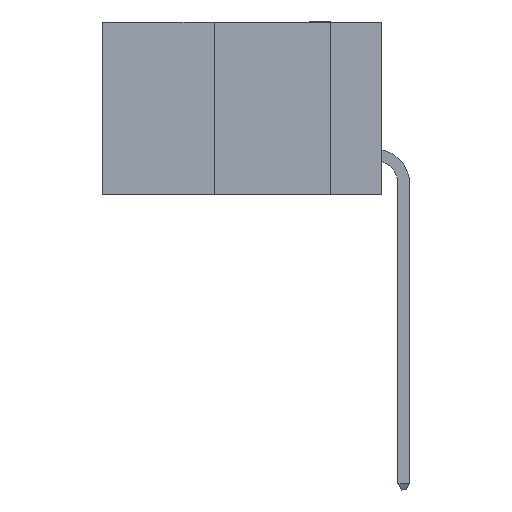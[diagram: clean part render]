
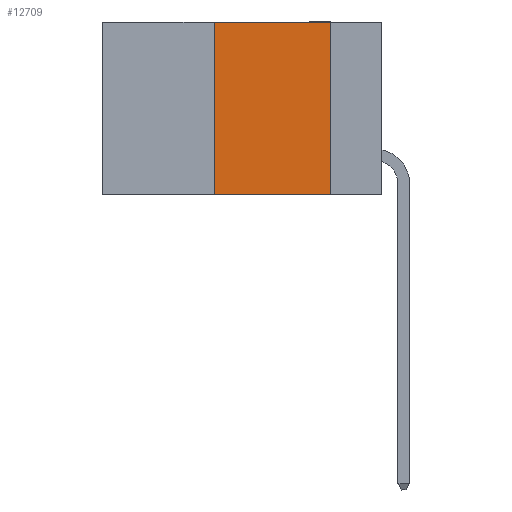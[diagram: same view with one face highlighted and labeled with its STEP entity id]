
A CAD part, left-side view. The second image highlights one B-rep face of the part: STEP entity #12709.
In plain terms, the highlighted planar face has unit normal (-1, 0, 0).
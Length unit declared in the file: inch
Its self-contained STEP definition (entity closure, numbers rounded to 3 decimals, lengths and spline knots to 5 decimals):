
#1251 = DIRECTION ( 'NONE',  ( 0., 0., -1. ) ) ;
#2239 = CARTESIAN_POINT ( 'NONE',  ( 0., 0.36, 0. ) ) ;
#2741 = DIRECTION ( 'NONE',  ( 1., 0., 0. ) ) ;
#4065 = CARTESIAN_POINT ( 'NONE',  ( 0., 0.11, 0. ) ) ;
#4241 = DIRECTION ( 'NONE',  ( 0., 0., 1. ) ) ;
#4516 = VERTEX_POINT ( 'NONE', #2239 ) ;
#4524 = ORIENTED_EDGE ( 'NONE', *, *, #6573, .F. ) ;
#4601 = EDGE_LOOP ( 'NONE', ( #8562, #8149, #4524, #5804 ) ) ;
#5652 = EDGE_CURVE ( 'NONE', #10325, #14951, #13583, .T. ) ;
#5702 = CARTESIAN_POINT ( 'NONE',  ( 0., 0.36, -0.37 ) ) ;
#5804 = ORIENTED_EDGE ( 'NONE', *, *, #5652, .T. ) ;
#5971 = LINE ( 'NONE', #6928, #12711 ) ;
#6346 = CARTESIAN_POINT ( 'NONE',  ( 0., 0.6, -0.37 ) ) ;
#6573 = EDGE_CURVE ( 'NONE', #10325, #4516, #5971, .T. ) ;
#6602 = EDGE_CURVE ( 'NONE', #4516, #11436, #8714, .T. ) ;
#6928 = CARTESIAN_POINT ( 'NONE',  ( 0., 0.36, 0. ) ) ;
#8149 = ORIENTED_EDGE ( 'NONE', *, *, #6602, .F. ) ;
#8562 = ORIENTED_EDGE ( 'NONE', *, *, #10153, .F. ) ;
#8714 = LINE ( 'NONE', #13705, #15413 ) ;
#9518 = CARTESIAN_POINT ( 'NONE',  ( 0., 0.6, 0. ) ) ;
#9568 = CARTESIAN_POINT ( 'NONE',  ( 0., 0.11, 0. ) ) ;
#10153 = EDGE_CURVE ( 'NONE', #11436, #14951, #14255, .T. ) ;
#10325 = VERTEX_POINT ( 'NONE', #5702 ) ;
#10873 = PLANE ( 'NONE',  #13644 ) ;
#11436 = VERTEX_POINT ( 'NONE', #9568 ) ;
#12225 = DIRECTION ( 'NONE',  ( 0., 0., -1. ) ) ;
#12709 = ADVANCED_FACE ( 'NONE', ( #17170 ), #10873, .F. ) ;
#12711 = VECTOR ( 'NONE', #4241, 39.37008 ) ;
#13583 = LINE ( 'NONE', #6346, #13986 ) ;
#13644 = AXIS2_PLACEMENT_3D ( 'NONE', #9518, #2741, #12225 ) ;
#13705 = CARTESIAN_POINT ( 'NONE',  ( 0., 0.6, 0. ) ) ;
#13986 = VECTOR ( 'NONE', #14379, 39.37008 ) ;
#14255 = LINE ( 'NONE', #4065, #17361 ) ;
#14379 = DIRECTION ( 'NONE',  ( 0., -1., 0. ) ) ;
#14951 = VERTEX_POINT ( 'NONE', #15822 ) ;
#15043 = DIRECTION ( 'NONE',  ( 0., -1., 0. ) ) ;
#15413 = VECTOR ( 'NONE', #15043, 39.37008 ) ;
#15822 = CARTESIAN_POINT ( 'NONE',  ( 0., 0.11, -0.37 ) ) ;
#17170 = FACE_OUTER_BOUND ( 'NONE', #4601, .T. ) ;
#17361 = VECTOR ( 'NONE', #1251, 39.37008 ) ;
